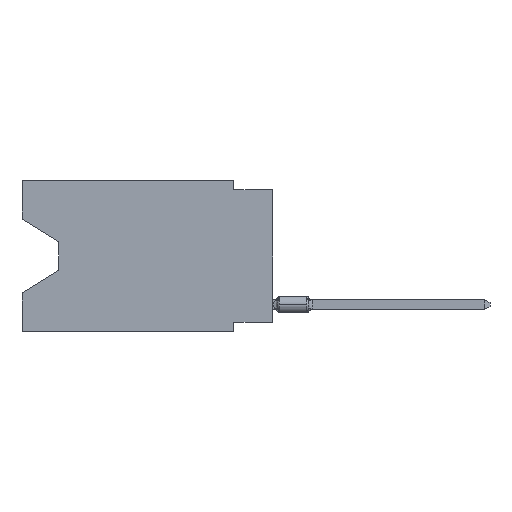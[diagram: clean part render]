
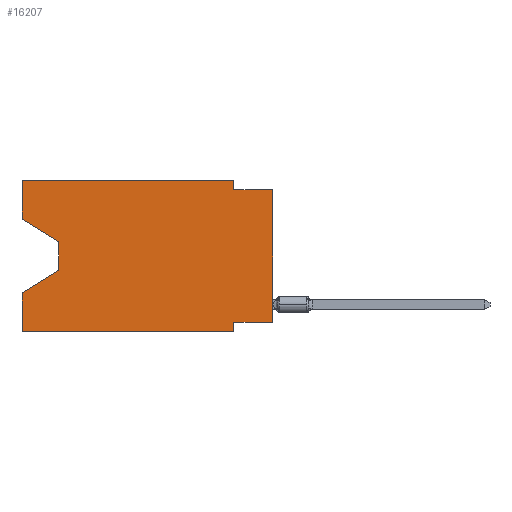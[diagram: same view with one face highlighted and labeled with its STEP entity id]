
A CAD part, left-side view. The second image highlights one B-rep face of the part: STEP entity #16207.
In plain terms, the highlighted planar face has unit normal (-1, 0, 0).
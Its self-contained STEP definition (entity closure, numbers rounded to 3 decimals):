
#115 = EDGE_LOOP ( 'NONE', ( #10499, #8295, #26281, #20585, #1269, #24279, #19823, #16282, #5906, #19468, #17982, #25896 ) ) ;
#264 = EDGE_CURVE ( 'NONE', #13041, #22208, #20903, .T. ) ;
#399 = LINE ( 'NONE', #8974, #14080 ) ;
#772 = DIRECTION ( 'NONE',  ( 0., -1., 0. ) ) ;
#1269 = ORIENTED_EDGE ( 'NONE', *, *, #9873, .T. ) ;
#1458 = DIRECTION ( 'NONE',  ( 0., 0., -1. ) ) ;
#1677 = VECTOR ( 'NONE', #772, 1000. ) ;
#2284 = CARTESIAN_POINT ( 'NONE',  ( 0., 0., -9.271 ) ) ;
#2668 = DIRECTION ( 'NONE',  ( 0., 0., -1. ) ) ;
#2717 = VERTEX_POINT ( 'NONE', #20711 ) ;
#2806 = EDGE_CURVE ( 'NONE', #25588, #22893, #12097, .T. ) ;
#3307 = DIRECTION ( 'NONE',  ( 0., 0., -1. ) ) ;
#3407 = CARTESIAN_POINT ( 'NONE',  ( 0., 0., -0.635 ) ) ;
#4000 = LINE ( 'NONE', #17261, #16443 ) ;
#4362 = FACE_OUTER_BOUND ( 'NONE', #115, .T. ) ;
#4792 = EDGE_CURVE ( 'NONE', #6064, #11232, #16133, .T. ) ;
#4824 = VERTEX_POINT ( 'NONE', #16548 ) ;
#5458 = LINE ( 'NONE', #13644, #9603 ) ;
#5906 = ORIENTED_EDGE ( 'NONE', *, *, #8377, .F. ) ;
#6064 = VERTEX_POINT ( 'NONE', #27245 ) ;
#6085 = CARTESIAN_POINT ( 'NONE',  ( 0., 2.54, -9.906 ) ) ;
#6831 = VERTEX_POINT ( 'NONE', #13484 ) ;
#7001 = VECTOR ( 'NONE', #24756, 1000. ) ;
#7187 = DIRECTION ( 'NONE',  ( 0., -1., 0. ) ) ;
#7381 = LINE ( 'NONE', #15988, #7001 ) ;
#7426 = CARTESIAN_POINT ( 'NONE',  ( 0., 16.383, 0. ) ) ;
#8295 = ORIENTED_EDGE ( 'NONE', *, *, #26501, .T. ) ;
#8377 = EDGE_CURVE ( 'NONE', #11232, #19715, #14005, .T. ) ;
#8974 = CARTESIAN_POINT ( 'NONE',  ( 0., 0., -9.271 ) ) ;
#8997 = DIRECTION ( 'NONE',  ( 1., 0., 0. ) ) ;
#9138 = PLANE ( 'NONE',  #20348 ) ;
#9162 = CARTESIAN_POINT ( 'NONE',  ( 0., 16.383, -9.906 ) ) ;
#9603 = VECTOR ( 'NONE', #15898, 1000. ) ;
#9710 = LINE ( 'NONE', #9162, #12369 ) ;
#9873 = EDGE_CURVE ( 'NONE', #11911, #22208, #9710, .T. ) ;
#10128 = VECTOR ( 'NONE', #22396, 1000. ) ;
#10499 = ORIENTED_EDGE ( 'NONE', *, *, #26979, .T. ) ;
#11232 = VERTEX_POINT ( 'NONE', #19868 ) ;
#11379 = CARTESIAN_POINT ( 'NONE',  ( 0., 2.54, -9.271 ) ) ;
#11814 = DIRECTION ( 'NONE',  ( 0., 0., 1. ) ) ;
#11911 = VERTEX_POINT ( 'NONE', #22935 ) ;
#11924 = LINE ( 'NONE', #25206, #10128 ) ;
#11973 = VECTOR ( 'NONE', #11814, 1000. ) ;
#12097 = LINE ( 'NONE', #16749, #11973 ) ;
#12369 = VECTOR ( 'NONE', #7187, 1000. ) ;
#12571 = CARTESIAN_POINT ( 'NONE',  ( 0., 0., 0. ) ) ;
#12602 = DIRECTION ( 'NONE',  ( 0., 0.855, -0.519 ) ) ;
#13041 = VERTEX_POINT ( 'NONE', #11379 ) ;
#13484 = CARTESIAN_POINT ( 'NONE',  ( 0., 16.383, -7.36 ) ) ;
#13487 = DIRECTION ( 'NONE',  ( 0., 1., 0. ) ) ;
#13644 = CARTESIAN_POINT ( 'NONE',  ( 0., 16.383, 0. ) ) ;
#14005 = LINE ( 'NONE', #24193, #1677 ) ;
#14080 = VECTOR ( 'NONE', #13487, 1000. ) ;
#15898 = DIRECTION ( 'NONE',  ( 0., 0., 1. ) ) ;
#15988 = CARTESIAN_POINT ( 'NONE',  ( 0., 16.383, -2.546 ) ) ;
#16039 = DIRECTION ( 'NONE',  ( 0., -1., 0. ) ) ;
#16133 = LINE ( 'NONE', #22918, #18764 ) ;
#16207 = ADVANCED_FACE ( 'NONE', ( #4362 ), #9138, .F. ) ;
#16282 = ORIENTED_EDGE ( 'NONE', *, *, #21806, .T. ) ;
#16359 = EDGE_CURVE ( 'NONE', #22893, #6064, #26502, .T. ) ;
#16443 = VECTOR ( 'NONE', #12602, 1000. ) ;
#16548 = CARTESIAN_POINT ( 'NONE',  ( 0., 13.97, -5.893 ) ) ;
#16749 = CARTESIAN_POINT ( 'NONE',  ( 0., 16.383, 0. ) ) ;
#17261 = CARTESIAN_POINT ( 'NONE',  ( 0., 13.97, -5.893 ) ) ;
#17539 = EDGE_CURVE ( 'NONE', #21935, #13041, #399, .T. ) ;
#17982 = ORIENTED_EDGE ( 'NONE', *, *, #16359, .F. ) ;
#18413 = CARTESIAN_POINT ( 'NONE',  ( 0., 16.383, 0. ) ) ;
#18764 = VECTOR ( 'NONE', #3307, 1000. ) ;
#18993 = VECTOR ( 'NONE', #16039, 1000. ) ;
#19468 = ORIENTED_EDGE ( 'NONE', *, *, #4792, .F. ) ;
#19715 = VERTEX_POINT ( 'NONE', #3407 ) ;
#19823 = ORIENTED_EDGE ( 'NONE', *, *, #17539, .F. ) ;
#19868 = CARTESIAN_POINT ( 'NONE',  ( 0., 2.54, -0.635 ) ) ;
#20348 = AXIS2_PLACEMENT_3D ( 'NONE', #21586, #8997, #2668 ) ;
#20585 = ORIENTED_EDGE ( 'NONE', *, *, #22361, .F. ) ;
#20711 = CARTESIAN_POINT ( 'NONE',  ( 0., 13.97, -4.013 ) ) ;
#20903 = LINE ( 'NONE', #6085, #21550 ) ;
#21305 = EDGE_CURVE ( 'NONE', #4824, #6831, #4000, .T. ) ;
#21550 = VECTOR ( 'NONE', #1458, 1000. ) ;
#21586 = CARTESIAN_POINT ( 'NONE',  ( 0., 16.383, 0. ) ) ;
#21780 = VECTOR ( 'NONE', #23161, 1000. ) ;
#21806 = EDGE_CURVE ( 'NONE', #21935, #19715, #27390, .T. ) ;
#21935 = VERTEX_POINT ( 'NONE', #2284 ) ;
#22208 = VERTEX_POINT ( 'NONE', #26094 ) ;
#22361 = EDGE_CURVE ( 'NONE', #11911, #6831, #5458, .T. ) ;
#22396 = DIRECTION ( 'NONE',  ( 0., 0., -1. ) ) ;
#22893 = VERTEX_POINT ( 'NONE', #18413 ) ;
#22918 = CARTESIAN_POINT ( 'NONE',  ( 0., 2.54, 0. ) ) ;
#22935 = CARTESIAN_POINT ( 'NONE',  ( 0., 16.383, -9.906 ) ) ;
#23161 = DIRECTION ( 'NONE',  ( 0., 0., 1. ) ) ;
#24193 = CARTESIAN_POINT ( 'NONE',  ( 0., 0., -0.635 ) ) ;
#24279 = ORIENTED_EDGE ( 'NONE', *, *, #264, .F. ) ;
#24756 = DIRECTION ( 'NONE',  ( 0., -0.855, -0.519 ) ) ;
#25206 = CARTESIAN_POINT ( 'NONE',  ( 0., 13.97, -4.013 ) ) ;
#25583 = CARTESIAN_POINT ( 'NONE',  ( 0., 16.383, -2.546 ) ) ;
#25588 = VERTEX_POINT ( 'NONE', #25583 ) ;
#25896 = ORIENTED_EDGE ( 'NONE', *, *, #2806, .F. ) ;
#26094 = CARTESIAN_POINT ( 'NONE',  ( 0., 2.54, -9.906 ) ) ;
#26281 = ORIENTED_EDGE ( 'NONE', *, *, #21305, .T. ) ;
#26501 = EDGE_CURVE ( 'NONE', #2717, #4824, #11924, .T. ) ;
#26502 = LINE ( 'NONE', #7426, #18993 ) ;
#26979 = EDGE_CURVE ( 'NONE', #25588, #2717, #7381, .T. ) ;
#27245 = CARTESIAN_POINT ( 'NONE',  ( 0., 2.54, 0. ) ) ;
#27390 = LINE ( 'NONE', #12571, #21780 ) ;
